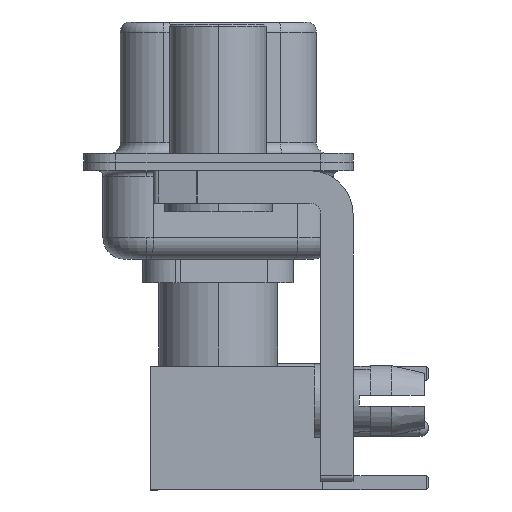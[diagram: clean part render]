
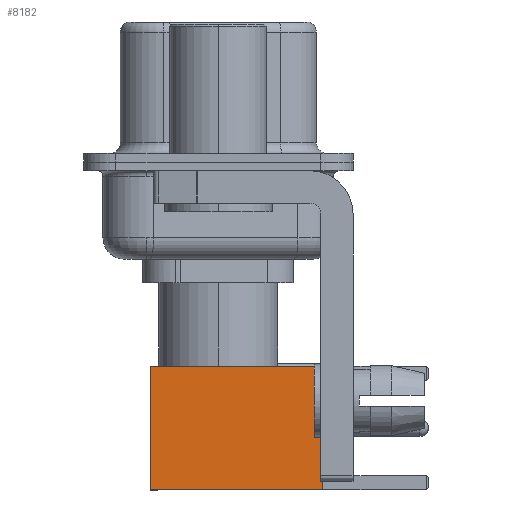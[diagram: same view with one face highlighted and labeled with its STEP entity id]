
A CAD part, left-side view. The second image highlights one B-rep face of the part: STEP entity #8182.
In plain terms, the highlighted face is planar.
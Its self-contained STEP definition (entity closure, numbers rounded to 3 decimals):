
#589 = CARTESIAN_POINT ( 'NONE',  ( 2.875, 2.875, 8. ) ) ;
#1539 = CARTESIAN_POINT ( 'NONE',  ( -2.875, 2.875, 0. ) ) ;
#2704 = DIRECTION ( 'NONE',  ( 0., 0., -1. ) ) ;
#4348 = LINE ( 'NONE', #21515, #20097 ) ;
#4812 = VERTEX_POINT ( 'NONE', #22819 ) ;
#5321 = ORIENTED_EDGE ( 'NONE', *, *, #10303, .F. ) ;
#5541 = VECTOR ( 'NONE', #9576, 1000. ) ;
#6052 = DIRECTION ( 'NONE',  ( 0., 1., 0. ) ) ;
#6457 = EDGE_CURVE ( 'NONE', #4812, #6734, #27158, .T. ) ;
#6734 = VERTEX_POINT ( 'NONE', #1539 ) ;
#8182 = ADVANCED_FACE ( 'NONE', ( #28038 ), #28604, .T. ) ;
#8426 = VECTOR ( 'NONE', #17867, 1000. ) ;
#9266 = ORIENTED_EDGE ( 'NONE', *, *, #18779, .T. ) ;
#9576 = DIRECTION ( 'NONE',  ( 0., 0., -1. ) ) ;
#9723 = CARTESIAN_POINT ( 'NONE',  ( 2.875, 2.875, 0. ) ) ;
#10303 = EDGE_CURVE ( 'NONE', #18898, #4812, #4348, .T. ) ;
#12580 = CARTESIAN_POINT ( 'NONE',  ( 2.875, 2.875, 0. ) ) ;
#13498 = LINE ( 'NONE', #27045, #8426 ) ;
#15065 = DIRECTION ( 'NONE',  ( 0., 0., 1. ) ) ;
#15792 = CARTESIAN_POINT ( 'NONE',  ( -2.875, 2.875, 0. ) ) ;
#15866 = CARTESIAN_POINT ( 'NONE',  ( 2.875, 2.875, 0. ) ) ;
#17867 = DIRECTION ( 'NONE',  ( -1., 0., 0. ) ) ;
#18779 = EDGE_CURVE ( 'NONE', #18898, #23607, #25596, .T. ) ;
#18898 = VERTEX_POINT ( 'NONE', #589 ) ;
#20097 = VECTOR ( 'NONE', #23993, 1000. ) ;
#20816 = EDGE_CURVE ( 'NONE', #23607, #6734, #13498, .T. ) ;
#21515 = CARTESIAN_POINT ( 'NONE',  ( 0., 2.875, 8. ) ) ;
#22819 = CARTESIAN_POINT ( 'NONE',  ( -2.875, 2.875, 8. ) ) ;
#23405 = EDGE_LOOP ( 'NONE', ( #9266, #24638, #25747, #5321 ) ) ;
#23607 = VERTEX_POINT ( 'NONE', #15866 ) ;
#23993 = DIRECTION ( 'NONE',  ( -1., 0., 0. ) ) ;
#24228 = AXIS2_PLACEMENT_3D ( 'NONE', #12580, #6052, #15065 ) ;
#24638 = ORIENTED_EDGE ( 'NONE', *, *, #20816, .T. ) ;
#25596 = LINE ( 'NONE', #9723, #5541 ) ;
#25747 = ORIENTED_EDGE ( 'NONE', *, *, #6457, .F. ) ;
#26918 = VECTOR ( 'NONE', #2704, 1000. ) ;
#27045 = CARTESIAN_POINT ( 'NONE',  ( 0., 2.875, 0. ) ) ;
#27158 = LINE ( 'NONE', #15792, #26918 ) ;
#28038 = FACE_OUTER_BOUND ( 'NONE', #23405, .T. ) ;
#28604 = PLANE ( 'NONE',  #24228 ) ;
